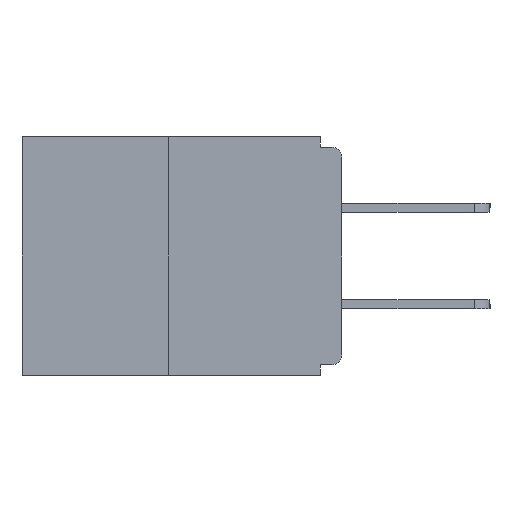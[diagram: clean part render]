
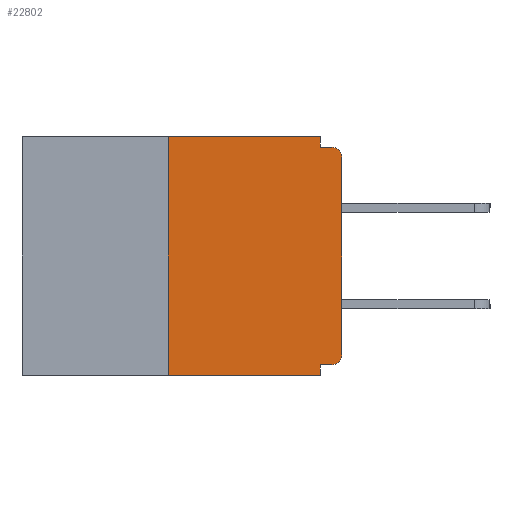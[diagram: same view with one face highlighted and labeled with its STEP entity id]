
A CAD part, left-side view. The second image highlights one B-rep face of the part: STEP entity #22802.
In plain terms, the highlighted planar face has unit normal (-1, 0, 0).
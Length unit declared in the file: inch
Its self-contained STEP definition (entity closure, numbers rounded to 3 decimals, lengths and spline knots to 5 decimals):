
#76 = CARTESIAN_POINT ( 'NONE',  ( 0., 0.46, 0. ) ) ;
#92 = VECTOR ( 'NONE', #18125, 39.37008 ) ;
#369 = DIRECTION ( 'NONE',  ( 0., 0., -1. ) ) ;
#730 = LINE ( 'NONE', #16694, #9330 ) ;
#868 = DIRECTION ( 'NONE',  ( 0., 0., -1. ) ) ;
#918 = CARTESIAN_POINT ( 'NONE',  ( 0., 0., -0.328 ) ) ;
#1377 = LINE ( 'NONE', #918, #15346 ) ;
#1460 = ORIENTED_EDGE ( 'NONE', *, *, #12707, .F. ) ;
#1488 = ORIENTED_EDGE ( 'NONE', *, *, #20977, .F. ) ;
#1730 = LINE ( 'NONE', #12150, #18374 ) ;
#1980 = DIRECTION ( 'NONE',  ( 1., 0., 0. ) ) ;
#2263 = CARTESIAN_POINT ( 'NONE',  ( 0., 0.015, -0.313 ) ) ;
#2549 = VECTOR ( 'NONE', #8620, 39.37008 ) ;
#2758 = CIRCLE ( 'NONE', #20791, 0.015 ) ;
#3065 = FACE_OUTER_BOUND ( 'NONE', #13372, .T. ) ;
#3762 = DIRECTION ( 'NONE',  ( 0., 0., 1. ) ) ;
#3775 = PLANE ( 'NONE',  #12410 ) ;
#4133 = CARTESIAN_POINT ( 'NONE',  ( 0., 0.031, -0.343 ) ) ;
#4610 = ORIENTED_EDGE ( 'NONE', *, *, #7702, .T. ) ;
#4726 = DIRECTION ( 'NONE',  ( 0., 1., 0. ) ) ;
#5028 = VERTEX_POINT ( 'NONE', #15600 ) ;
#5219 = EDGE_CURVE ( 'NONE', #24426, #24592, #18526, .T. ) ;
#5625 = LINE ( 'NONE', #18758, #22874 ) ;
#5842 = LINE ( 'NONE', #13254, #2549 ) ;
#5959 = DIRECTION ( 'NONE',  ( 0., 0., -1. ) ) ;
#5977 = VERTEX_POINT ( 'NONE', #12196 ) ;
#6244 = ORIENTED_EDGE ( 'NONE', *, *, #15431, .T. ) ;
#6816 = EDGE_CURVE ( 'NONE', #24426, #14327, #12764, .T. ) ;
#7221 = CARTESIAN_POINT ( 'NONE',  ( 0., 0.031, -0.328 ) ) ;
#7356 = VERTEX_POINT ( 'NONE', #9477 ) ;
#7702 = EDGE_CURVE ( 'NONE', #7356, #13255, #21387, .T. ) ;
#8433 = CARTESIAN_POINT ( 'NONE',  ( 0., 0.015, -0.03 ) ) ;
#8620 = DIRECTION ( 'NONE',  ( 0., 0., -1. ) ) ;
#8722 = CARTESIAN_POINT ( 'NONE',  ( 0., 0.031, 0. ) ) ;
#9330 = VECTOR ( 'NONE', #3762, 39.37008 ) ;
#9403 = DIRECTION ( 'NONE',  ( 0., -1., 0. ) ) ;
#9477 = CARTESIAN_POINT ( 'NONE',  ( 0., 0.015, -0.328 ) ) ;
#10347 = DIRECTION ( 'NONE',  ( -1., 0., 0. ) ) ;
#11198 = DIRECTION ( 'NONE',  ( 0., -1., 0. ) ) ;
#11662 = VECTOR ( 'NONE', #9403, 39.37008 ) ;
#11829 = CARTESIAN_POINT ( 'NONE',  ( 0., 0.015, -0.015 ) ) ;
#12150 = CARTESIAN_POINT ( 'NONE',  ( 0., 0.46, 0. ) ) ;
#12196 = CARTESIAN_POINT ( 'NONE',  ( 0., 0.031, -0.015 ) ) ;
#12410 = AXIS2_PLACEMENT_3D ( 'NONE', #76, #1980, #5959 ) ;
#12552 = LINE ( 'NONE', #8722, #92 ) ;
#12707 = EDGE_CURVE ( 'NONE', #14327, #15066, #1730, .T. ) ;
#12764 = LINE ( 'NONE', #13272, #23193 ) ;
#13254 = CARTESIAN_POINT ( 'NONE',  ( 0., 0.031, -0.343 ) ) ;
#13255 = VERTEX_POINT ( 'NONE', #18175 ) ;
#13272 = CARTESIAN_POINT ( 'NONE',  ( 0., 0.25, 0. ) ) ;
#13372 = EDGE_LOOP ( 'NONE', ( #1460, #22620, #20576, #1488, #19911, #4610, #17212, #6244, #18171, #22959 ) ) ;
#13515 = DIRECTION ( 'NONE',  ( -1., 0., 0. ) ) ;
#13804 = EDGE_CURVE ( 'NONE', #7356, #15036, #1377, .T. ) ;
#14327 = VERTEX_POINT ( 'NONE', #23031 ) ;
#15036 = VERTEX_POINT ( 'NONE', #7221 ) ;
#15066 = VERTEX_POINT ( 'NONE', #16812 ) ;
#15230 = DIRECTION ( 'NONE',  ( 0., -1., 0. ) ) ;
#15346 = VECTOR ( 'NONE', #4726, 39.37008 ) ;
#15379 = CARTESIAN_POINT ( 'NONE',  ( 0., 0.46, -0.343 ) ) ;
#15431 = EDGE_CURVE ( 'NONE', #5028, #18142, #2758, .T. ) ;
#15600 = CARTESIAN_POINT ( 'NONE',  ( 0., 0., -0.03 ) ) ;
#16191 = AXIS2_PLACEMENT_3D ( 'NONE', #2263, #13515, #369 ) ;
#16694 = CARTESIAN_POINT ( 'NONE',  ( 0., 0., 0. ) ) ;
#16812 = CARTESIAN_POINT ( 'NONE',  ( 0., 0.031, 0. ) ) ;
#17212 = ORIENTED_EDGE ( 'NONE', *, *, #17624, .T. ) ;
#17624 = EDGE_CURVE ( 'NONE', #13255, #5028, #730, .T. ) ;
#17808 = EDGE_CURVE ( 'NONE', #15066, #5977, #12552, .T. ) ;
#18125 = DIRECTION ( 'NONE',  ( 0., 0., -1. ) ) ;
#18142 = VERTEX_POINT ( 'NONE', #11829 ) ;
#18171 = ORIENTED_EDGE ( 'NONE', *, *, #19720, .F. ) ;
#18175 = CARTESIAN_POINT ( 'NONE',  ( 0., 0., -0.313 ) ) ;
#18374 = VECTOR ( 'NONE', #15230, 39.37008 ) ;
#18526 = LINE ( 'NONE', #15379, #11662 ) ;
#18758 = CARTESIAN_POINT ( 'NONE',  ( 0., 0., -0.015 ) ) ;
#19720 = EDGE_CURVE ( 'NONE', #5977, #18142, #5625, .T. ) ;
#19911 = ORIENTED_EDGE ( 'NONE', *, *, #13804, .F. ) ;
#20576 = ORIENTED_EDGE ( 'NONE', *, *, #5219, .T. ) ;
#20791 = AXIS2_PLACEMENT_3D ( 'NONE', #8433, #10347, #868 ) ;
#20977 = EDGE_CURVE ( 'NONE', #15036, #24592, #5842, .T. ) ;
#21387 = CIRCLE ( 'NONE', #16191, 0.015 ) ;
#22575 = DIRECTION ( 'NONE',  ( 0., 0., 1. ) ) ;
#22620 = ORIENTED_EDGE ( 'NONE', *, *, #6816, .F. ) ;
#22802 = ADVANCED_FACE ( 'NONE', ( #3065 ), #3775, .F. ) ;
#22874 = VECTOR ( 'NONE', #11198, 39.37008 ) ;
#22959 = ORIENTED_EDGE ( 'NONE', *, *, #17808, .F. ) ;
#23031 = CARTESIAN_POINT ( 'NONE',  ( 0., 0.25, 0. ) ) ;
#23193 = VECTOR ( 'NONE', #22575, 39.37008 ) ;
#24426 = VERTEX_POINT ( 'NONE', #24567 ) ;
#24567 = CARTESIAN_POINT ( 'NONE',  ( 0., 0.25, -0.343 ) ) ;
#24592 = VERTEX_POINT ( 'NONE', #4133 ) ;
